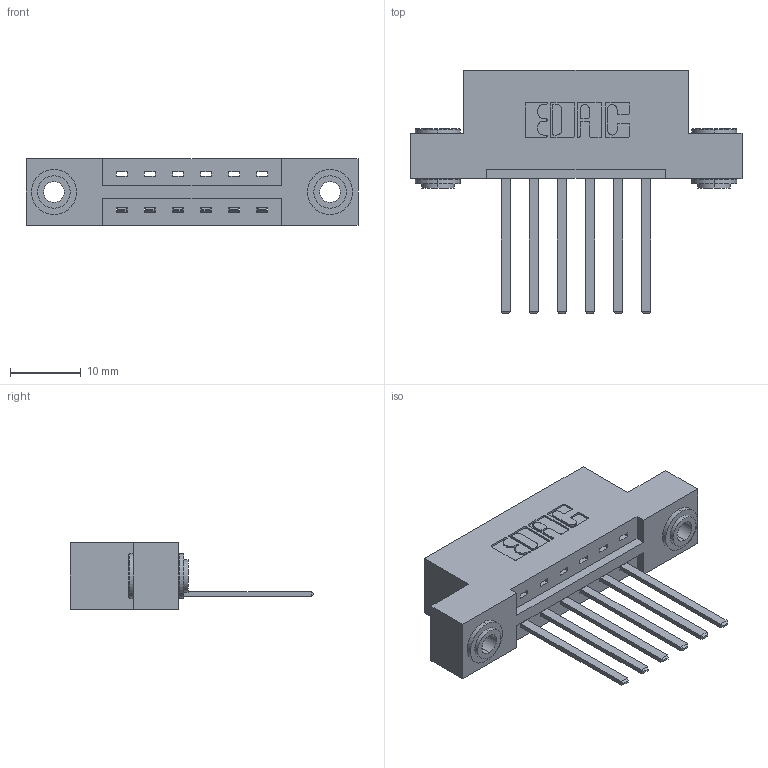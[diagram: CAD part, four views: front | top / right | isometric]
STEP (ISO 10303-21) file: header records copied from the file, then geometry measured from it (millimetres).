
FILE_DESCRIPTION (( 'STEP AP203' ), '1' );
FILE_NAME ('337-006-544-103.STEP', '2019-09-27T17:18:32', ( '' ), ( '' ), 'SwSTEP 2.0', 'SolidWorks 2016', '' );
FILE_SCHEMA (( 'CONFIG_CONTROL_DESIGN' ));
Length unit declared in the file: inch
Products named in the file (4): 337-006-544-103; 345-292-001_345-293-144; 337 Part_Flush Mounting Lugs - 0.156 Dia-TH; 345-250-002_345-250-002-102
Assembly tree (9 placements, depth 2):
  337-006-544-103
    337 Part_Flush Mounting Lugs - 0.156 Dia-TH
    345-292-001_345-293-144  x6
    345-250-002_345-250-002-102  x2
Bounding box: 46.79 x 34.3 x 9.4 mm (x, y, z)
Volume: 4501.1 mm3; surface area: 4912.7 mm2
Topology: 9 solids, 9 shells, 488 faces, 1407 edges, 926 vertices
Faces by surface type: plane 332, cylinder 148, cone 8
Entity records: 9582 total; most frequent: CARTESIAN_POINT 1643, ORIENTED_EDGE 1578, DIRECTION 1487, EDGE_CURVE 789, VECTOR 641, LINE 641, VERTEX_POINT 522, AXIS2_PLACEMENT_3D 423
